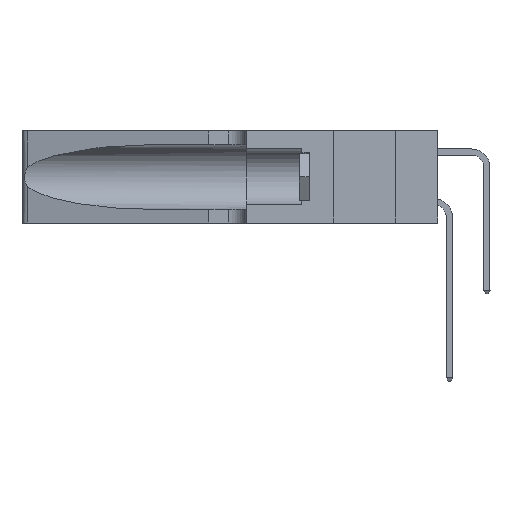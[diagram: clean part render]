
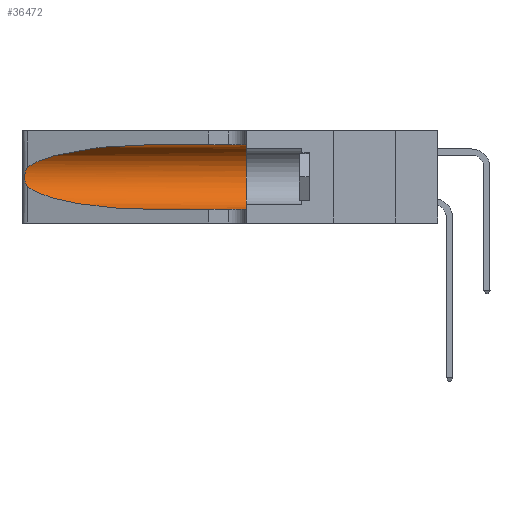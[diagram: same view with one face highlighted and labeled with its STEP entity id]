
A CAD part, left-side view. The second image highlights one B-rep face of the part: STEP entity #36472.
In plain terms, the highlighted cylindrical face has radius 3.308 mm (diameter 6.617 mm), a partial arc.
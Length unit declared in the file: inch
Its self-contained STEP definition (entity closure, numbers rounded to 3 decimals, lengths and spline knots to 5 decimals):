
#331 = DIRECTION ( 'NONE',  ( 0., -1., 0. ) ) ;
#407 = ORIENTED_EDGE ( 'NONE', *, *, #8505, .T. ) ;
#428 = CARTESIAN_POINT ( 'NONE',  ( 0.25487, 1.22718, 0.14631 ) ) ;
#461 = CIRCLE ( 'NONE', #44184, 0.13025 ) ;
#1322 = LINE ( 'NONE', #2749, #38592 ) ;
#1473 = CYLINDRICAL_SURFACE ( 'NONE', #31250, 0.13025 ) ;
#1877 = ORIENTED_EDGE ( 'NONE', *, *, #22831, .F. ) ;
#2179 = ORIENTED_EDGE ( 'NONE', *, *, #32179, .T. ) ;
#2256 =( BOUNDED_CURVE ( )  B_SPLINE_CURVE ( 3, ( #23931, #44820, #6503, #30974 ),
 .UNSPECIFIED., .F., .F. ) 
 B_SPLINE_CURVE_WITH_KNOTS ( ( 4, 4 ),
 ( 1.5708, 2.84003 ),
 .UNSPECIFIED. ) 
 CURVE ( )  GEOMETRIC_REPRESENTATION_ITEM ( )  RATIONAL_B_SPLINE_CURVE ( ( 1., 0.87, 0.87, 1. ) ) 
 REPRESENTATION_ITEM ( '' )  );
#2749 = CARTESIAN_POINT ( 'NONE',  ( 0.1305, 1.61858, 0.05475 ) ) ;
#3008 = CARTESIAN_POINT ( 'NONE',  ( 0.1305, 0.35, 0.185 ) ) ;
#3271 = CARTESIAN_POINT ( 'NONE',  ( 0.1305, 0.72297, 0.05475 ) ) ;
#3756 = FACE_OUTER_BOUND ( 'NONE', #35050, .T. ) ;
#3928 = CARTESIAN_POINT ( 'NONE',  ( 0.25487, 1.22718, 0.22369 ) ) ;
#3990 = DIRECTION ( 'NONE',  ( 0., 0., -1. ) ) ;
#4638 = VECTOR ( 'NONE', #26447, 39.37008 ) ;
#5344 = CARTESIAN_POINT ( 'NONE',  ( 0.1305, 1.61858, 0.31525 ) ) ;
#6503 = CARTESIAN_POINT ( 'NONE',  ( 0.2373, 1.15595, 0.28018 ) ) ;
#6520 = DIRECTION ( 'NONE',  ( 0., 0., 1. ) ) ;
#7192 = CARTESIAN_POINT ( 'NONE',  ( 0.1305, 0.35, 0.31525 ) ) ;
#7449 = CARTESIAN_POINT ( 'NONE',  ( 0.25854, 1.2359, 0.20912 ) ) ;
#8505 = EDGE_CURVE ( 'NONE', #19450, #9928, #26676, .T. ) ;
#9928 = VERTEX_POINT ( 'NONE', #25297 ) ;
#10948 = CARTESIAN_POINT ( 'NONE',  ( 0.26075, 1.23896, 0.19203 ) ) ;
#11949 = CARTESIAN_POINT ( 'NONE',  ( 0.1305, 0.72297, 0.31525 ) ) ;
#13145 = DIRECTION ( 'NONE',  ( 0., -1., 0. ) ) ;
#13654 = CARTESIAN_POINT ( 'NONE',  ( 0.2373, 1.15595, 0.08982 ) ) ;
#13658 = VERTEX_POINT ( 'NONE', #29839 ) ;
#14318 = CARTESIAN_POINT ( 'NONE',  ( 0.25639, 1.23184, 0.21858 ) ) ;
#14470 = CARTESIAN_POINT ( 'NONE',  ( 0.26017, 1.23833, 0.17102 ) ) ;
#14615 = VERTEX_POINT ( 'NONE', #20626 ) ;
#17129 = EDGE_CURVE ( 'NONE', #43201, #13658, #461, .T. ) ;
#17973 = CARTESIAN_POINT ( 'NONE',  ( 0.25789, 1.23486, 0.15765 ) ) ;
#19450 = VERTEX_POINT ( 'NONE', #20816 ) ;
#20626 = CARTESIAN_POINT ( 'NONE',  ( 0.1305, 0.72297, 0.05475 ) ) ;
#20816 = CARTESIAN_POINT ( 'NONE',  ( 0.25487, 1.22718, 0.22369 ) ) ;
#21543 = CARTESIAN_POINT ( 'NONE',  ( 0.25555, 1.22993, 0.14849 ) ) ;
#22831 = EDGE_CURVE ( 'NONE', #28601, #43201, #23228, .T. ) ;
#23228 = LINE ( 'NONE', #5344, #4638 ) ;
#23679 = EDGE_CURVE ( 'NONE', #28601, #19450, #2256, .T. ) ;
#23931 = CARTESIAN_POINT ( 'NONE',  ( 0.1305, 0.72297, 0.31525 ) ) ;
#24213 = CARTESIAN_POINT ( 'NONE',  ( 0.18966, 0.96281, 0.05475 ) ) ;
#25297 = CARTESIAN_POINT ( 'NONE',  ( 0.25487, 1.22718, 0.14631 ) ) ;
#26447 = DIRECTION ( 'NONE',  ( 0., -1., 0. ) ) ;
#26676 = B_SPLINE_CURVE_WITH_KNOTS ( 'NONE', 3,
 ( #3928, #38755, #14318, #28381, #7449, #31886, #10948, #35400, #14470, #38912, #17973, #42415, #21543, #428 ),
 .UNSPECIFIED., .F., .F.,
 ( 4, 2, 2, 2, 2, 2, 4 ),
 ( 0., 0.00027, 0.00053, 0.00107, 0.0016, 0.00187, 0.00214 ),
 .UNSPECIFIED. ) ;
#27479 = DIRECTION ( 'NONE',  ( 0., 1., 0. ) ) ;
#28381 = CARTESIAN_POINT ( 'NONE',  ( 0.25787, 1.23484, 0.2124 ) ) ;
#28601 = VERTEX_POINT ( 'NONE', #11949 ) ;
#28975 = ORIENTED_EDGE ( 'NONE', *, *, #37936, .T. ) ;
#29839 = CARTESIAN_POINT ( 'NONE',  ( 0.1305, 0.35, 0.05475 ) ) ;
#30974 = CARTESIAN_POINT ( 'NONE',  ( 0.25487, 1.22718, 0.22369 ) ) ;
#31250 = AXIS2_PLACEMENT_3D ( 'NONE', #31795, #331, #3990 ) ;
#31795 = CARTESIAN_POINT ( 'NONE',  ( 0.1305, 1.61858, 0.185 ) ) ;
#31886 = CARTESIAN_POINT ( 'NONE',  ( 0.26018, 1.23835, 0.19895 ) ) ;
#32179 = EDGE_CURVE ( 'NONE', #14615, #13658, #1322, .T. ) ;
#35050 = EDGE_LOOP ( 'NONE', ( #42801, #407, #28975, #2179, #45343, #1877 ) ) ;
#35400 = CARTESIAN_POINT ( 'NONE',  ( 0.26075, 1.23896, 0.178 ) ) ;
#36205 =( BOUNDED_CURVE ( )  B_SPLINE_CURVE ( 3, ( #38105, #13654, #24213, #3271 ),
 .UNSPECIFIED., .F., .F. ) 
 B_SPLINE_CURVE_WITH_KNOTS ( ( 4, 4 ),
 ( 3.44316, 4.71239 ),
 .UNSPECIFIED. ) 
 CURVE ( )  GEOMETRIC_REPRESENTATION_ITEM ( )  RATIONAL_B_SPLINE_CURVE ( ( 1., 0.87, 0.87, 1. ) ) 
 REPRESENTATION_ITEM ( '' )  );
#36472 = ADVANCED_FACE ( 'NONE', ( #3756 ), #1473, .F. ) ;
#37936 = EDGE_CURVE ( 'NONE', #9928, #14615, #36205, .T. ) ;
#38105 = CARTESIAN_POINT ( 'NONE',  ( 0.25487, 1.22718, 0.14631 ) ) ;
#38592 = VECTOR ( 'NONE', #13145, 39.37008 ) ;
#38755 = CARTESIAN_POINT ( 'NONE',  ( 0.25555, 1.22994, 0.2215 ) ) ;
#38912 = CARTESIAN_POINT ( 'NONE',  ( 0.25856, 1.23593, 0.16098 ) ) ;
#42415 = CARTESIAN_POINT ( 'NONE',  ( 0.25639, 1.23186, 0.15144 ) ) ;
#42801 = ORIENTED_EDGE ( 'NONE', *, *, #23679, .T. ) ;
#43201 = VERTEX_POINT ( 'NONE', #7192 ) ;
#44184 = AXIS2_PLACEMENT_3D ( 'NONE', #3008, #27479, #6520 ) ;
#44820 = CARTESIAN_POINT ( 'NONE',  ( 0.18966, 0.96281, 0.31525 ) ) ;
#45343 = ORIENTED_EDGE ( 'NONE', *, *, #17129, .F. ) ;
